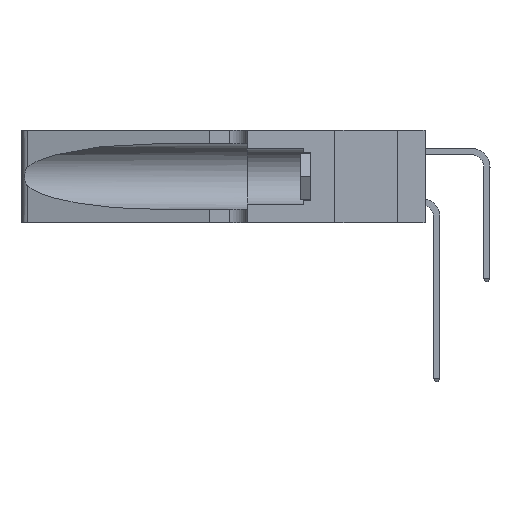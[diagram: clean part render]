
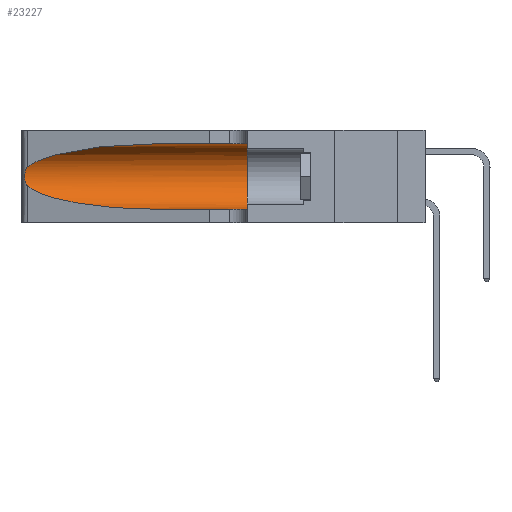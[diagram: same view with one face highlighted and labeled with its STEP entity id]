
A CAD part, left-side view. The second image highlights one B-rep face of the part: STEP entity #23227.
In plain terms, the highlighted cylindrical face has radius 3.308 mm (diameter 6.617 mm), a partial arc.
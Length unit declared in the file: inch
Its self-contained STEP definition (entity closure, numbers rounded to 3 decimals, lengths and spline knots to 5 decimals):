
#737 = EDGE_CURVE ( 'NONE', #32797, #4064, #22722, .T. ) ;
#792 = VERTEX_POINT ( 'NONE', #21094 ) ;
#1018 = ORIENTED_EDGE ( 'NONE', *, *, #1098, .T. ) ;
#1098 = EDGE_CURVE ( 'NONE', #14690, #792, #12406, .T. ) ;
#1938 = CARTESIAN_POINT ( 'NONE',  ( 0.25639, 1.23186, 0.15144 ) ) ;
#2285 = AXIS2_PLACEMENT_3D ( 'NONE', #23277, #6431, #34188 ) ;
#2876 = ORIENTED_EDGE ( 'NONE', *, *, #34221, .T. ) ;
#4064 = VERTEX_POINT ( 'NONE', #34662 ) ;
#4557 = VECTOR ( 'NONE', #27942, 39.37008 ) ;
#4846 = CARTESIAN_POINT ( 'NONE',  ( 0.25487, 1.22718, 0.14631 ) ) ;
#6431 = DIRECTION ( 'NONE',  ( 0., -1., 0. ) ) ;
#6653 = CYLINDRICAL_SURFACE ( 'NONE', #2285, 0.13025 ) ;
#7577 = CARTESIAN_POINT ( 'NONE',  ( 0.25639, 1.23184, 0.21858 ) ) ;
#8422 = CARTESIAN_POINT ( 'NONE',  ( 0.1305, 0.35, 0.31525 ) ) ;
#10175 = CARTESIAN_POINT ( 'NONE',  ( 0.1305, 0.72297, 0.31525 ) ) ;
#10399 = CARTESIAN_POINT ( 'NONE',  ( 0.25854, 1.2359, 0.20912 ) ) ;
#11969 = CARTESIAN_POINT ( 'NONE',  ( 0.1305, 0.72297, 0.05475 ) ) ;
#12406 =( BOUNDED_CURVE ( )  B_SPLINE_CURVE ( 3, ( #19359, #24927, #30461, #13779 ),
 .UNSPECIFIED., .F., .F. ) 
 B_SPLINE_CURVE_WITH_KNOTS ( ( 4, 4 ),
 ( 1.5708, 2.84003 ),
 .UNSPECIFIED. ) 
 CURVE ( )  GEOMETRIC_REPRESENTATION_ITEM ( )  RATIONAL_B_SPLINE_CURVE ( ( 1., 0.87, 0.87, 1. ) ) 
 REPRESENTATION_ITEM ( '' )  );
#13201 = CARTESIAN_POINT ( 'NONE',  ( 0.26075, 1.23896, 0.19203 ) ) ;
#13459 = VECTOR ( 'NONE', #23342, 39.37008 ) ;
#13779 = CARTESIAN_POINT ( 'NONE',  ( 0.25487, 1.22718, 0.22369 ) ) ;
#14690 = VERTEX_POINT ( 'NONE', #10175 ) ;
#15194 = CARTESIAN_POINT ( 'NONE',  ( 0.1305, 0.35, 0.185 ) ) ;
#15257 = CARTESIAN_POINT ( 'NONE',  ( 0.18966, 0.96281, 0.05475 ) ) ;
#16087 = CARTESIAN_POINT ( 'NONE',  ( 0.26017, 1.23833, 0.17102 ) ) ;
#16371 = EDGE_LOOP ( 'NONE', ( #1018, #23608, #2876, #25306, #27037, #20572 ) ) ;
#18041 = DIRECTION ( 'NONE',  ( 0., 0., 1. ) ) ;
#18805 = CARTESIAN_POINT ( 'NONE',  ( 0.25555, 1.22994, 0.2215 ) ) ;
#18923 = CARTESIAN_POINT ( 'NONE',  ( 0.25789, 1.23486, 0.15765 ) ) ;
#19359 = CARTESIAN_POINT ( 'NONE',  ( 0.1305, 0.72297, 0.31525 ) ) ;
#19557 = LINE ( 'NONE', #25167, #4557 ) ;
#19681 = EDGE_CURVE ( 'NONE', #792, #33939, #26508, .T. ) ;
#20559 = CARTESIAN_POINT ( 'NONE',  ( 0.1305, 1.61858, 0.05475 ) ) ;
#20572 = ORIENTED_EDGE ( 'NONE', *, *, #21755, .F. ) ;
#21094 = CARTESIAN_POINT ( 'NONE',  ( 0.25487, 1.22718, 0.22369 ) ) ;
#21739 = CARTESIAN_POINT ( 'NONE',  ( 0.25555, 1.22993, 0.14849 ) ) ;
#21755 = EDGE_CURVE ( 'NONE', #14690, #32797, #19557, .T. ) ;
#22722 = CIRCLE ( 'NONE', #27950, 0.13025 ) ;
#23227 = ADVANCED_FACE ( 'NONE', ( #31514 ), #6653, .F. ) ;
#23277 = CARTESIAN_POINT ( 'NONE',  ( 0.1305, 1.61858, 0.185 ) ) ;
#23342 = DIRECTION ( 'NONE',  ( 0., -1., 0. ) ) ;
#23579 = CARTESIAN_POINT ( 'NONE',  ( 0.2373, 1.15595, 0.08982 ) ) ;
#23608 = ORIENTED_EDGE ( 'NONE', *, *, #19681, .T. ) ;
#23895 =( BOUNDED_CURVE ( )  B_SPLINE_CURVE ( 3, ( #26308, #23579, #15257, #34604 ),
 .UNSPECIFIED., .F., .F. ) 
 B_SPLINE_CURVE_WITH_KNOTS ( ( 4, 4 ),
 ( 3.44316, 4.71239 ),
 .UNSPECIFIED. ) 
 CURVE ( )  GEOMETRIC_REPRESENTATION_ITEM ( )  RATIONAL_B_SPLINE_CURVE ( ( 1., 0.87, 0.87, 1. ) ) 
 REPRESENTATION_ITEM ( '' )  );
#24927 = CARTESIAN_POINT ( 'NONE',  ( 0.18966, 0.96281, 0.31525 ) ) ;
#25167 = CARTESIAN_POINT ( 'NONE',  ( 0.1305, 1.61858, 0.31525 ) ) ;
#25306 = ORIENTED_EDGE ( 'NONE', *, *, #29645, .T. ) ;
#26308 = CARTESIAN_POINT ( 'NONE',  ( 0.25487, 1.22718, 0.14631 ) ) ;
#26508 = B_SPLINE_CURVE_WITH_KNOTS ( 'NONE', 3,
 ( #35296, #18805, #7577, #27130, #10399, #29922, #13201, #32671, #16087, #35418, #18923, #1938, #21739, #4846 ),
 .UNSPECIFIED., .F., .F.,
 ( 4, 2, 2, 2, 2, 2, 4 ),
 ( 0., 0.00027, 0.00053, 0.00107, 0.0016, 0.00187, 0.00214 ),
 .UNSPECIFIED. ) ;
#27037 = ORIENTED_EDGE ( 'NONE', *, *, #737, .F. ) ;
#27130 = CARTESIAN_POINT ( 'NONE',  ( 0.25787, 1.23484, 0.2124 ) ) ;
#27942 = DIRECTION ( 'NONE',  ( 0., -1., 0. ) ) ;
#27950 = AXIS2_PLACEMENT_3D ( 'NONE', #15194, #34542, #18041 ) ;
#29645 = EDGE_CURVE ( 'NONE', #34803, #4064, #35593, .T. ) ;
#29922 = CARTESIAN_POINT ( 'NONE',  ( 0.26018, 1.23835, 0.19895 ) ) ;
#30461 = CARTESIAN_POINT ( 'NONE',  ( 0.2373, 1.15595, 0.28018 ) ) ;
#31514 = FACE_OUTER_BOUND ( 'NONE', #16371, .T. ) ;
#32671 = CARTESIAN_POINT ( 'NONE',  ( 0.26075, 1.23896, 0.178 ) ) ;
#32797 = VERTEX_POINT ( 'NONE', #8422 ) ;
#33939 = VERTEX_POINT ( 'NONE', #36073 ) ;
#34188 = DIRECTION ( 'NONE',  ( 0., 0., -1. ) ) ;
#34221 = EDGE_CURVE ( 'NONE', #33939, #34803, #23895, .T. ) ;
#34542 = DIRECTION ( 'NONE',  ( 0., 1., 0. ) ) ;
#34604 = CARTESIAN_POINT ( 'NONE',  ( 0.1305, 0.72297, 0.05475 ) ) ;
#34662 = CARTESIAN_POINT ( 'NONE',  ( 0.1305, 0.35, 0.05475 ) ) ;
#34803 = VERTEX_POINT ( 'NONE', #11969 ) ;
#35296 = CARTESIAN_POINT ( 'NONE',  ( 0.25487, 1.22718, 0.22369 ) ) ;
#35418 = CARTESIAN_POINT ( 'NONE',  ( 0.25856, 1.23593, 0.16098 ) ) ;
#35593 = LINE ( 'NONE', #20559, #13459 ) ;
#36073 = CARTESIAN_POINT ( 'NONE',  ( 0.25487, 1.22718, 0.14631 ) ) ;
